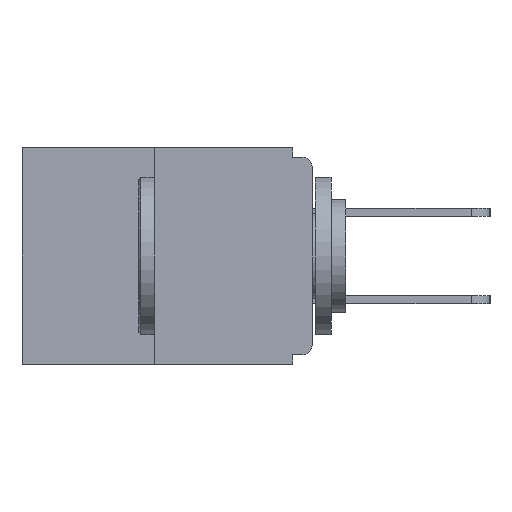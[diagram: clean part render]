
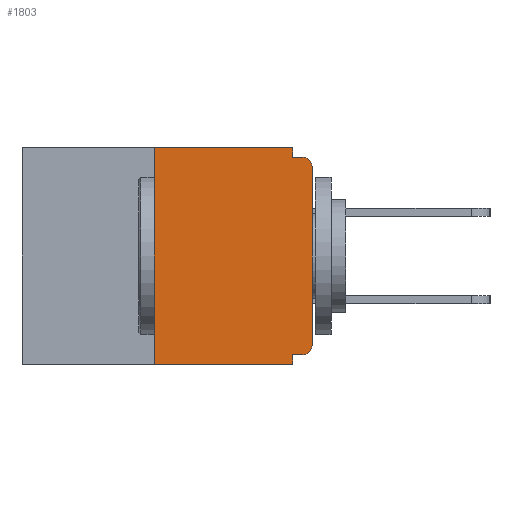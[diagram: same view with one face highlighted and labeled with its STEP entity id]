
A CAD part, left-side view. The second image highlights one B-rep face of the part: STEP entity #1803.
In plain terms, the highlighted planar face has unit normal (-1, 0, 0).
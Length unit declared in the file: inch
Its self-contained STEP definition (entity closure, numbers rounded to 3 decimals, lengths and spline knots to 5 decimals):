
#352 = CIRCLE ( 'NONE', #1535, 0.015 ) ;
#1278 = ORIENTED_EDGE ( 'NONE', *, *, #3456, .F. ) ;
#1329 = VERTEX_POINT ( 'NONE', #11124 ) ;
#1535 = AXIS2_PLACEMENT_3D ( 'NONE', #14784, #5647, #10138 ) ;
#1687 = CARTESIAN_POINT ( 'NONE',  ( 0., 0., -0.03 ) ) ;
#1740 = LINE ( 'NONE', #4367, #2442 ) ;
#1795 = EDGE_CURVE ( 'NONE', #1329, #9528, #1740, .T. ) ;
#1803 = ADVANCED_FACE ( 'NONE', ( #8027 ), #5719, .F. ) ;
#2258 = CARTESIAN_POINT ( 'NONE',  ( 0., 0.031, 0. ) ) ;
#2442 = VECTOR ( 'NONE', #4559, 39.37008 ) ;
#2479 = EDGE_CURVE ( 'NONE', #8904, #10185, #11545, .T. ) ;
#2548 = ORIENTED_EDGE ( 'NONE', *, *, #8642, .F. ) ;
#2564 = EDGE_LOOP ( 'NONE', ( #10639, #3183, #5613, #2548, #1278, #12911, #4641, #10411, #12942, #4138 ) ) ;
#2750 = LINE ( 'NONE', #4652, #11186 ) ;
#2865 = VECTOR ( 'NONE', #5010, 39.37008 ) ;
#2990 = EDGE_CURVE ( 'NONE', #8227, #6917, #4532, .T. ) ;
#3021 = DIRECTION ( 'NONE',  ( 0., 0., -1. ) ) ;
#3183 = ORIENTED_EDGE ( 'NONE', *, *, #10556, .F. ) ;
#3312 = CARTESIAN_POINT ( 'NONE',  ( 0., 0.46, 0. ) ) ;
#3456 = EDGE_CURVE ( 'NONE', #10071, #9937, #2750, .T. ) ;
#3562 = CARTESIAN_POINT ( 'NONE',  ( 0., 0.46, -0.343 ) ) ;
#3642 = VECTOR ( 'NONE', #12477, 39.37008 ) ;
#4138 = ORIENTED_EDGE ( 'NONE', *, *, #2990, .F. ) ;
#4367 = CARTESIAN_POINT ( 'NONE',  ( 0., 0., 0. ) ) ;
#4532 = LINE ( 'NONE', #2258, #3642 ) ;
#4559 = DIRECTION ( 'NONE',  ( 0., 0., 1. ) ) ;
#4641 = ORIENTED_EDGE ( 'NONE', *, *, #1795, .T. ) ;
#4652 = CARTESIAN_POINT ( 'NONE',  ( 0., 0., -0.328 ) ) ;
#4721 = DIRECTION ( 'NONE',  ( 0., -1., 0. ) ) ;
#5010 = DIRECTION ( 'NONE',  ( 0., 0., 1. ) ) ;
#5053 = CIRCLE ( 'NONE', #9278, 0.015 ) ;
#5107 = CARTESIAN_POINT ( 'NONE',  ( 0., 0.25, 0. ) ) ;
#5132 = VECTOR ( 'NONE', #14392, 39.37008 ) ;
#5595 = EDGE_CURVE ( 'NONE', #5952, #8227, #11663, .T. ) ;
#5613 = ORIENTED_EDGE ( 'NONE', *, *, #2479, .T. ) ;
#5647 = DIRECTION ( 'NONE',  ( -1., 0., 0. ) ) ;
#5719 = PLANE ( 'NONE',  #6563 ) ;
#5819 = CARTESIAN_POINT ( 'NONE',  ( 0., 0.031, -0.328 ) ) ;
#5952 = VERTEX_POINT ( 'NONE', #5107 ) ;
#6156 = CARTESIAN_POINT ( 'NONE',  ( 0., 0.031, -0.343 ) ) ;
#6173 = CARTESIAN_POINT ( 'NONE',  ( 0., 0.25, 0. ) ) ;
#6284 = LINE ( 'NONE', #6173, #2865 ) ;
#6551 = EDGE_CURVE ( 'NONE', #6917, #8960, #11964, .T. ) ;
#6563 = AXIS2_PLACEMENT_3D ( 'NONE', #3312, #12553, #8067 ) ;
#6636 = CARTESIAN_POINT ( 'NONE',  ( 0., 0.031, -0.343 ) ) ;
#6917 = VERTEX_POINT ( 'NONE', #10232 ) ;
#8014 = VECTOR ( 'NONE', #4721, 39.37008 ) ;
#8027 = FACE_OUTER_BOUND ( 'NONE', #2564, .T. ) ;
#8067 = DIRECTION ( 'NONE',  ( 0., 0., -1. ) ) ;
#8227 = VERTEX_POINT ( 'NONE', #11546 ) ;
#8349 = CARTESIAN_POINT ( 'NONE',  ( 0., 0.25, -0.343 ) ) ;
#8642 = EDGE_CURVE ( 'NONE', #9937, #10185, #12087, .T. ) ;
#8885 = DIRECTION ( 'NONE',  ( 0., 0., -1. ) ) ;
#8904 = VERTEX_POINT ( 'NONE', #8349 ) ;
#8960 = VERTEX_POINT ( 'NONE', #14220 ) ;
#9278 = AXIS2_PLACEMENT_3D ( 'NONE', #9921, #12116, #3021 ) ;
#9528 = VERTEX_POINT ( 'NONE', #1687 ) ;
#9843 = CARTESIAN_POINT ( 'NONE',  ( 0., 0.015, -0.328 ) ) ;
#9921 = CARTESIAN_POINT ( 'NONE',  ( 0., 0.015, -0.03 ) ) ;
#9937 = VERTEX_POINT ( 'NONE', #5819 ) ;
#10071 = VERTEX_POINT ( 'NONE', #9843 ) ;
#10138 = DIRECTION ( 'NONE',  ( 0., 0., -1. ) ) ;
#10185 = VERTEX_POINT ( 'NONE', #6156 ) ;
#10232 = CARTESIAN_POINT ( 'NONE',  ( 0., 0.031, -0.015 ) ) ;
#10411 = ORIENTED_EDGE ( 'NONE', *, *, #14573, .T. ) ;
#10556 = EDGE_CURVE ( 'NONE', #8904, #5952, #6284, .T. ) ;
#10613 = EDGE_CURVE ( 'NONE', #10071, #1329, #352, .T. ) ;
#10615 = VECTOR ( 'NONE', #11159, 39.37008 ) ;
#10639 = ORIENTED_EDGE ( 'NONE', *, *, #5595, .F. ) ;
#10648 = VECTOR ( 'NONE', #8885, 39.37008 ) ;
#11124 = CARTESIAN_POINT ( 'NONE',  ( 0., 0., -0.313 ) ) ;
#11159 = DIRECTION ( 'NONE',  ( 0., -1., 0. ) ) ;
#11186 = VECTOR ( 'NONE', #13825, 39.37008 ) ;
#11545 = LINE ( 'NONE', #3562, #8014 ) ;
#11546 = CARTESIAN_POINT ( 'NONE',  ( 0., 0.031, 0. ) ) ;
#11663 = LINE ( 'NONE', #14362, #10615 ) ;
#11964 = LINE ( 'NONE', #12091, #5132 ) ;
#12087 = LINE ( 'NONE', #6636, #10648 ) ;
#12091 = CARTESIAN_POINT ( 'NONE',  ( 0., 0., -0.015 ) ) ;
#12116 = DIRECTION ( 'NONE',  ( -1., 0., 0. ) ) ;
#12477 = DIRECTION ( 'NONE',  ( 0., 0., -1. ) ) ;
#12553 = DIRECTION ( 'NONE',  ( 1., 0., 0. ) ) ;
#12911 = ORIENTED_EDGE ( 'NONE', *, *, #10613, .T. ) ;
#12942 = ORIENTED_EDGE ( 'NONE', *, *, #6551, .F. ) ;
#13825 = DIRECTION ( 'NONE',  ( 0., 1., 0. ) ) ;
#14220 = CARTESIAN_POINT ( 'NONE',  ( 0., 0.015, -0.015 ) ) ;
#14362 = CARTESIAN_POINT ( 'NONE',  ( 0., 0.46, 0. ) ) ;
#14392 = DIRECTION ( 'NONE',  ( 0., -1., 0. ) ) ;
#14573 = EDGE_CURVE ( 'NONE', #9528, #8960, #5053, .T. ) ;
#14784 = CARTESIAN_POINT ( 'NONE',  ( 0., 0.015, -0.313 ) ) ;
